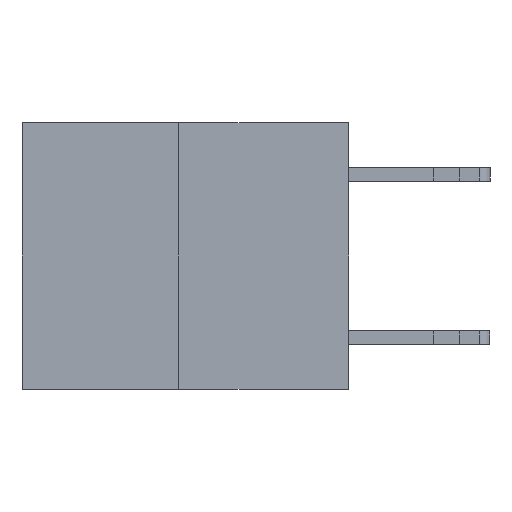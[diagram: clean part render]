
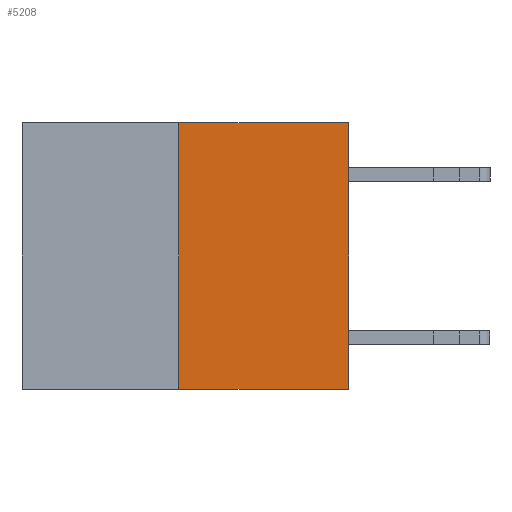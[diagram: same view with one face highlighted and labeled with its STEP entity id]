
A CAD part, left-side view. The second image highlights one B-rep face of the part: STEP entity #5208.
In plain terms, the highlighted planar face has unit normal (-1, 0, 0).
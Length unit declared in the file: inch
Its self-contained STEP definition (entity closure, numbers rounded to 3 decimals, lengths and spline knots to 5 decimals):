
#356 = VERTEX_POINT ( 'NONE', #6177 ) ;
#441 = VERTEX_POINT ( 'NONE', #11222 ) ;
#451 = FACE_OUTER_BOUND ( 'NONE', #12940, .T. ) ;
#909 = LINE ( 'NONE', #10036, #15255 ) ;
#1313 = EDGE_CURVE ( 'NONE', #11121, #441, #7072, .T. ) ;
#2797 = VECTOR ( 'NONE', #4669, 39.37008 ) ;
#2937 = ORIENTED_EDGE ( 'NONE', *, *, #8609, .T. ) ;
#3157 = PLANE ( 'NONE',  #6490 ) ;
#3221 = CARTESIAN_POINT ( 'NONE',  ( 0., 0.6, -0.49 ) ) ;
#3552 = DIRECTION ( 'NONE',  ( 1., 0., 0. ) ) ;
#4669 = DIRECTION ( 'NONE',  ( 0., -1., 0. ) ) ;
#4699 = LINE ( 'NONE', #3221, #18294 ) ;
#5208 = ADVANCED_FACE ( 'NONE', ( #451 ), #3157, .F. ) ;
#5215 = CARTESIAN_POINT ( 'NONE',  ( 0., 0., -0.49 ) ) ;
#5561 = ORIENTED_EDGE ( 'NONE', *, *, #19039, .F. ) ;
#6177 = CARTESIAN_POINT ( 'NONE',  ( 0., 0.312, -0.49 ) ) ;
#6288 = DIRECTION ( 'NONE',  ( 0., 0., 1. ) ) ;
#6490 = AXIS2_PLACEMENT_3D ( 'NONE', #19407, #3552, #15777 ) ;
#7072 = LINE ( 'NONE', #20320, #10567 ) ;
#8609 = EDGE_CURVE ( 'NONE', #356, #11121, #4699, .T. ) ;
#9913 = EDGE_CURVE ( 'NONE', #356, #13573, #909, .T. ) ;
#10036 = CARTESIAN_POINT ( 'NONE',  ( 0., 0.312, -0.49 ) ) ;
#10567 = VECTOR ( 'NONE', #6288, 39.37008 ) ;
#11121 = VERTEX_POINT ( 'NONE', #5215 ) ;
#11222 = CARTESIAN_POINT ( 'NONE',  ( 0., 0., 0. ) ) ;
#12457 = ORIENTED_EDGE ( 'NONE', *, *, #1313, .T. ) ;
#12940 = EDGE_LOOP ( 'NONE', ( #16945, #2937, #12457, #5561 ) ) ;
#13222 = DIRECTION ( 'NONE',  ( 0., 0., 1. ) ) ;
#13573 = VERTEX_POINT ( 'NONE', #14919 ) ;
#14919 = CARTESIAN_POINT ( 'NONE',  ( 0., 0.312, 0. ) ) ;
#15255 = VECTOR ( 'NONE', #13222, 39.37008 ) ;
#15777 = DIRECTION ( 'NONE',  ( 0., 0., -1. ) ) ;
#16945 = ORIENTED_EDGE ( 'NONE', *, *, #9913, .F. ) ;
#17431 = DIRECTION ( 'NONE',  ( 0., -1., 0. ) ) ;
#18294 = VECTOR ( 'NONE', #17431, 39.37008 ) ;
#18590 = LINE ( 'NONE', #18816, #2797 ) ;
#18816 = CARTESIAN_POINT ( 'NONE',  ( 0., 0.6, 0. ) ) ;
#19039 = EDGE_CURVE ( 'NONE', #13573, #441, #18590, .T. ) ;
#19407 = CARTESIAN_POINT ( 'NONE',  ( 0., 0.6, 0. ) ) ;
#20320 = CARTESIAN_POINT ( 'NONE',  ( 0., 0., 0. ) ) ;
